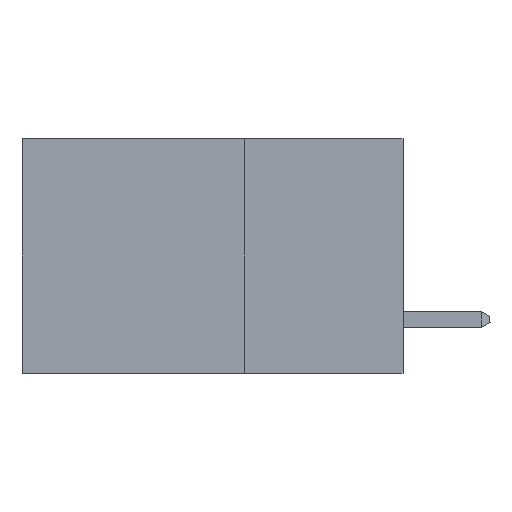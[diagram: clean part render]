
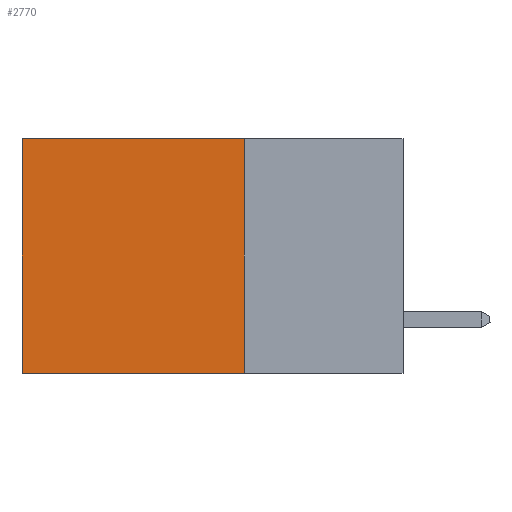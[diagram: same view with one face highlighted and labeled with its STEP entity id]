
A CAD part, left-side view. The second image highlights one B-rep face of the part: STEP entity #2770.
In plain terms, the highlighted planar face has unit normal (-1, 0, 0).
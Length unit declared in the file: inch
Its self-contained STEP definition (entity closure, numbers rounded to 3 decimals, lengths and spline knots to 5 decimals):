
#1217 = CARTESIAN_POINT ( 'NONE',  ( 0.2875, 0.25, -0.37 ) ) ;
#1357 = DIRECTION ( 'NONE',  ( 1., 0., 0. ) ) ;
#1465 = PLANE ( 'NONE',  #7600 ) ;
#1690 = ORIENTED_EDGE ( 'NONE', *, *, #10231, .T. ) ;
#1817 = VECTOR ( 'NONE', #15357, 39.37008 ) ;
#1851 = EDGE_LOOP ( 'NONE', ( #12366, #6478, #14787, #1690 ) ) ;
#2236 = CARTESIAN_POINT ( 'NONE',  ( 0.2875, 0.25, 0. ) ) ;
#2300 = CARTESIAN_POINT ( 'NONE',  ( 0.2875, 0.25, 0. ) ) ;
#2371 = LINE ( 'NONE', #9762, #5589 ) ;
#2488 = VERTEX_POINT ( 'NONE', #11564 ) ;
#2727 = DIRECTION ( 'NONE',  ( 0., 0., -1. ) ) ;
#2770 = ADVANCED_FACE ( 'NONE', ( #3575 ), #1465, .F. ) ;
#3575 = FACE_OUTER_BOUND ( 'NONE', #1851, .T. ) ;
#3848 = CARTESIAN_POINT ( 'NONE',  ( 0.2875, 0.25, 0. ) ) ;
#3933 = DIRECTION ( 'NONE',  ( 0., 1., 0. ) ) ;
#5589 = VECTOR ( 'NONE', #15144, 39.37008 ) ;
#5952 = LINE ( 'NONE', #2236, #1817 ) ;
#6478 = ORIENTED_EDGE ( 'NONE', *, *, #13655, .F. ) ;
#7600 = AXIS2_PLACEMENT_3D ( 'NONE', #3848, #1357, #2727 ) ;
#8379 = EDGE_CURVE ( 'NONE', #15238, #2488, #2371, .T. ) ;
#8719 = LINE ( 'NONE', #2300, #13554 ) ;
#8979 = EDGE_CURVE ( 'NONE', #11679, #13546, #5952, .T. ) ;
#9762 = CARTESIAN_POINT ( 'NONE',  ( 0.2875, 0.6, 0. ) ) ;
#10231 = EDGE_CURVE ( 'NONE', #11679, #15238, #8719, .T. ) ;
#11045 = CARTESIAN_POINT ( 'NONE',  ( 0.2875, 0.25, -0.37 ) ) ;
#11564 = CARTESIAN_POINT ( 'NONE',  ( 0.2875, 0.6, -0.37 ) ) ;
#11598 = CARTESIAN_POINT ( 'NONE',  ( 0.2875, 0.25, 0. ) ) ;
#11679 = VERTEX_POINT ( 'NONE', #11598 ) ;
#12283 = DIRECTION ( 'NONE',  ( 0., 1., 0. ) ) ;
#12366 = ORIENTED_EDGE ( 'NONE', *, *, #8379, .T. ) ;
#13204 = CARTESIAN_POINT ( 'NONE',  ( 0.2875, 0.6, 0. ) ) ;
#13546 = VERTEX_POINT ( 'NONE', #1217 ) ;
#13554 = VECTOR ( 'NONE', #3933, 39.37008 ) ;
#13655 = EDGE_CURVE ( 'NONE', #13546, #2488, #14261, .T. ) ;
#14261 = LINE ( 'NONE', #11045, #15209 ) ;
#14787 = ORIENTED_EDGE ( 'NONE', *, *, #8979, .F. ) ;
#15144 = DIRECTION ( 'NONE',  ( 0., 0., -1. ) ) ;
#15209 = VECTOR ( 'NONE', #12283, 39.37008 ) ;
#15238 = VERTEX_POINT ( 'NONE', #13204 ) ;
#15357 = DIRECTION ( 'NONE',  ( 0., 0., -1. ) ) ;
